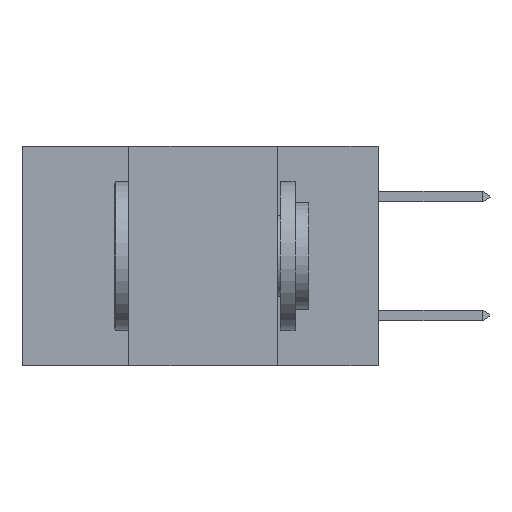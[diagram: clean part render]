
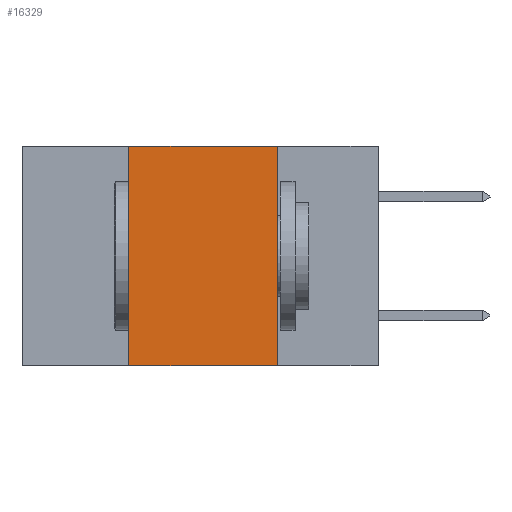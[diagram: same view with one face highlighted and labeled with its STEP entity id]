
A CAD part, left-side view. The second image highlights one B-rep face of the part: STEP entity #16329.
In plain terms, the highlighted planar face has unit normal (-1, 0, 0).
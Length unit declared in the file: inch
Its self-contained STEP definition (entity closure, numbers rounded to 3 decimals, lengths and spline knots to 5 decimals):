
#2690 = VECTOR ( 'NONE', #25033, 39.37008 ) ;
#5617 = CARTESIAN_POINT ( 'NONE',  ( 0., 0.17, 0. ) ) ;
#6068 = CARTESIAN_POINT ( 'NONE',  ( 0., 0.42, 0. ) ) ;
#7354 = LINE ( 'NONE', #30410, #25629 ) ;
#7597 = DIRECTION ( 'NONE',  ( 0., -1., 0. ) ) ;
#7818 = VECTOR ( 'NONE', #25394, 39.37008 ) ;
#7911 = CARTESIAN_POINT ( 'NONE',  ( 0., 0.42, -0.37 ) ) ;
#8739 = VERTEX_POINT ( 'NONE', #22929 ) ;
#9777 = AXIS2_PLACEMENT_3D ( 'NONE', #23729, #14321, #19115 ) ;
#10177 = LINE ( 'NONE', #5617, #2690 ) ;
#10358 = EDGE_CURVE ( 'NONE', #30488, #27777, #15804, .T. ) ;
#12581 = EDGE_CURVE ( 'NONE', #13015, #30488, #26866, .T. ) ;
#13015 = VERTEX_POINT ( 'NONE', #7911 ) ;
#13854 = CARTESIAN_POINT ( 'NONE',  ( 0., 0.17, 0. ) ) ;
#14321 = DIRECTION ( 'NONE',  ( 1., 0., 0. ) ) ;
#14799 = ORIENTED_EDGE ( 'NONE', *, *, #25456, .T. ) ;
#14922 = CARTESIAN_POINT ( 'NONE',  ( 0., 0.6, 0. ) ) ;
#15804 = LINE ( 'NONE', #14922, #24399 ) ;
#16329 = ADVANCED_FACE ( 'NONE', ( #17997 ), #23622, .F. ) ;
#17997 = FACE_OUTER_BOUND ( 'NONE', #19673, .T. ) ;
#18227 = ORIENTED_EDGE ( 'NONE', *, *, #26173, .F. ) ;
#19115 = DIRECTION ( 'NONE',  ( 0., 0., -1. ) ) ;
#19432 = ORIENTED_EDGE ( 'NONE', *, *, #10358, .F. ) ;
#19673 = EDGE_LOOP ( 'NONE', ( #18227, #19432, #27093, #14799 ) ) ;
#22929 = CARTESIAN_POINT ( 'NONE',  ( 0., 0.17, -0.37 ) ) ;
#23013 = DIRECTION ( 'NONE',  ( 0., -1., 0. ) ) ;
#23622 = PLANE ( 'NONE',  #9777 ) ;
#23729 = CARTESIAN_POINT ( 'NONE',  ( 0., 0.6, 0. ) ) ;
#24399 = VECTOR ( 'NONE', #7597, 39.37008 ) ;
#24515 = CARTESIAN_POINT ( 'NONE',  ( 0., 0.42, 0. ) ) ;
#25033 = DIRECTION ( 'NONE',  ( 0., 0., -1. ) ) ;
#25394 = DIRECTION ( 'NONE',  ( 0., 0., 1. ) ) ;
#25456 = EDGE_CURVE ( 'NONE', #13015, #8739, #7354, .T. ) ;
#25629 = VECTOR ( 'NONE', #23013, 39.37008 ) ;
#26173 = EDGE_CURVE ( 'NONE', #27777, #8739, #10177, .T. ) ;
#26866 = LINE ( 'NONE', #6068, #7818 ) ;
#27093 = ORIENTED_EDGE ( 'NONE', *, *, #12581, .F. ) ;
#27777 = VERTEX_POINT ( 'NONE', #13854 ) ;
#30410 = CARTESIAN_POINT ( 'NONE',  ( 0., 0.6, -0.37 ) ) ;
#30488 = VERTEX_POINT ( 'NONE', #24515 ) ;
